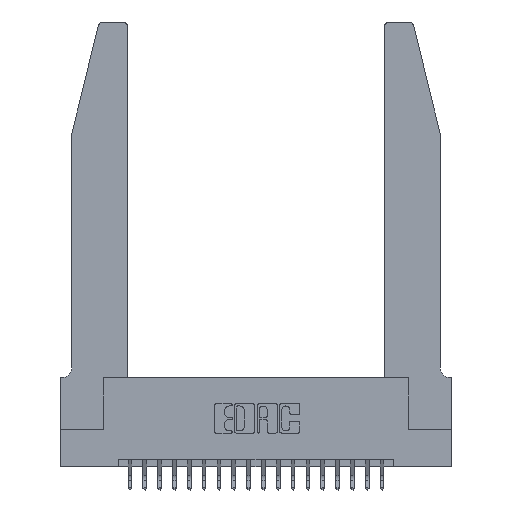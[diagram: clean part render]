
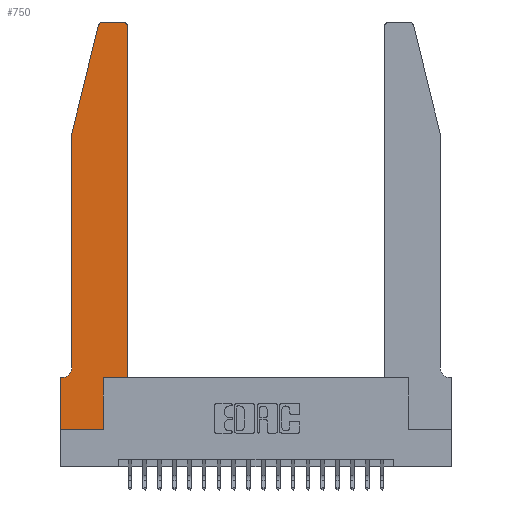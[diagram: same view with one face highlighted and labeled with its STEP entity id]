
A CAD part, top view. The second image highlights one B-rep face of the part: STEP entity #750.
In plain terms, the highlighted planar face has unit normal (0, 0, 1).
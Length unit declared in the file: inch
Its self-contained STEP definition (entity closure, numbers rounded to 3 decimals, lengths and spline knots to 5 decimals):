
#50 = VERTEX_POINT ( 'NONE', #18213 ) ;
#88 = ORIENTED_EDGE ( 'NONE', *, *, #21648, .T. ) ;
#132 = CARTESIAN_POINT ( 'NONE',  ( 0.2865, 0., 0.37 ) ) ;
#356 = LINE ( 'NONE', #10773, #19022 ) ;
#670 = CARTESIAN_POINT ( 'NONE',  ( 0.0755, 2., 0.37 ) ) ;
#750 = ADVANCED_FACE ( 'NONE', ( #14140 ), #21990, .T. ) ;
#799 = VERTEX_POINT ( 'NONE', #10004 ) ;
#1168 = LINE ( 'NONE', #1817, #9071 ) ;
#1387 = DIRECTION ( 'NONE',  ( 1., 0., 0. ) ) ;
#1817 = CARTESIAN_POINT ( 'NONE',  ( 0., 0., 0.37 ) ) ;
#1843 = CARTESIAN_POINT ( 'NONE',  ( 0.284, 2.75, 0.37 ) ) ;
#2261 = CIRCLE ( 'NONE', #8044, 0.03 ) ;
#2303 = VECTOR ( 'NONE', #19196, 39.37008 ) ;
#2811 = LINE ( 'NONE', #670, #19023 ) ;
#2984 = ORIENTED_EDGE ( 'NONE', *, *, #8302, .T. ) ;
#3949 = LINE ( 'NONE', #14047, #2303 ) ;
#4034 = DIRECTION ( 'NONE',  ( 1., 0., 0. ) ) ;
#4175 = CARTESIAN_POINT ( 'NONE',  ( 0., 0., 0.37 ) ) ;
#4612 = VERTEX_POINT ( 'NONE', #22006 ) ;
#4892 = EDGE_CURVE ( 'NONE', #15860, #11558, #11312, .T. ) ;
#5032 = ORIENTED_EDGE ( 'NONE', *, *, #19874, .T. ) ;
#5102 = EDGE_CURVE ( 'NONE', #50, #15860, #3949, .T. ) ;
#5191 = VECTOR ( 'NONE', #19702, 39.37008 ) ;
#5246 = CARTESIAN_POINT ( 'NONE',  ( 0.0755, 0.35, 0.37 ) ) ;
#5864 = LINE ( 'NONE', #14336, #19835 ) ;
#5895 = EDGE_CURVE ( 'NONE', #8026, #19718, #5864, .T. ) ;
#6040 = LINE ( 'NONE', #15882, #10870 ) ;
#6229 = EDGE_CURVE ( 'NONE', #10780, #50, #2261, .T. ) ;
#6900 = VERTEX_POINT ( 'NONE', #7355 ) ;
#7232 = CARTESIAN_POINT ( 'NONE',  ( 0.0055, 0.42, 0.37 ) ) ;
#7264 = CARTESIAN_POINT ( 'NONE',  ( 0., 0., 0.37 ) ) ;
#7355 = CARTESIAN_POINT ( 'NONE',  ( 0.0055, 0.35, 0.37 ) ) ;
#7405 = DIRECTION ( 'NONE',  ( 0., -1., 0. ) ) ;
#8026 = VERTEX_POINT ( 'NONE', #21622 ) ;
#8044 = AXIS2_PLACEMENT_3D ( 'NONE', #15621, #12115, #20733 ) ;
#8132 = LINE ( 'NONE', #7264, #21272 ) ;
#8302 = EDGE_CURVE ( 'NONE', #19718, #10780, #6040, .T. ) ;
#8345 = CARTESIAN_POINT ( 'NONE',  ( 0., 0.35, 0.37 ) ) ;
#8570 = LINE ( 'NONE', #5246, #20934 ) ;
#9071 = VECTOR ( 'NONE', #7405, 39.37008 ) ;
#9343 = CARTESIAN_POINT ( 'NONE',  ( 0.2865, 0.35, 0.37 ) ) ;
#10004 = CARTESIAN_POINT ( 'NONE',  ( 0.0755, 0.42, 0.37 ) ) ;
#10617 = ORIENTED_EDGE ( 'NONE', *, *, #4892, .T. ) ;
#10773 = CARTESIAN_POINT ( 'NONE',  ( 0.0755, 2., 0.37 ) ) ;
#10780 = VERTEX_POINT ( 'NONE', #20130 ) ;
#10870 = VECTOR ( 'NONE', #10917, 39.37008 ) ;
#10916 = DIRECTION ( 'NONE',  ( 0., 0., -1. ) ) ;
#10917 = DIRECTION ( 'NONE',  ( 0., 1., 0. ) ) ;
#10988 = DIRECTION ( 'NONE',  ( 0., -1., 0. ) ) ;
#11066 = ORIENTED_EDGE ( 'NONE', *, *, #14176, .T. ) ;
#11136 = CARTESIAN_POINT ( 'NONE',  ( 0.4505, 0.35, 0.37 ) ) ;
#11141 = LINE ( 'NONE', #9343, #5191 ) ;
#11235 = ORIENTED_EDGE ( 'NONE', *, *, #16200, .T. ) ;
#11312 = CIRCLE ( 'NONE', #20836, 0.03 ) ;
#11558 = VERTEX_POINT ( 'NONE', #15691 ) ;
#11735 = DIRECTION ( 'NONE',  ( 0., 0., 1. ) ) ;
#12115 = DIRECTION ( 'NONE',  ( 0., 0., 1. ) ) ;
#12174 = ORIENTED_EDGE ( 'NONE', *, *, #5102, .T. ) ;
#12661 = CARTESIAN_POINT ( 'NONE',  ( 0.284, 2.72, 0.37 ) ) ;
#12680 = EDGE_CURVE ( 'NONE', #799, #6900, #21186, .T. ) ;
#13039 = EDGE_CURVE ( 'NONE', #11558, #4612, #356, .T. ) ;
#13253 = EDGE_CURVE ( 'NONE', #14546, #18317, #1168, .T. ) ;
#13934 = AXIS2_PLACEMENT_3D ( 'NONE', #8345, #11735, #1387 ) ;
#14047 = CARTESIAN_POINT ( 'NONE',  ( 0.2605, 2.75, 0.37 ) ) ;
#14140 = FACE_OUTER_BOUND ( 'NONE', #17117, .T. ) ;
#14176 = EDGE_CURVE ( 'NONE', #4612, #799, #2811, .T. ) ;
#14185 = DIRECTION ( 'NONE',  ( 1., 0., 0. ) ) ;
#14336 = CARTESIAN_POINT ( 'NONE',  ( 0.4505, 0.35, 0.37 ) ) ;
#14401 = DIRECTION ( 'NONE',  ( 0., 0., 1. ) ) ;
#14546 = VERTEX_POINT ( 'NONE', #15054 ) ;
#15054 = CARTESIAN_POINT ( 'NONE',  ( 0., 0.35, 0.37 ) ) ;
#15621 = CARTESIAN_POINT ( 'NONE',  ( 0.4205, 2.72, 0.37 ) ) ;
#15691 = CARTESIAN_POINT ( 'NONE',  ( 0.25487, 2.72718, 0.37 ) ) ;
#15735 = DIRECTION ( 'NONE',  ( -0.239, -0.971, 0. ) ) ;
#15860 = VERTEX_POINT ( 'NONE', #1843 ) ;
#15882 = CARTESIAN_POINT ( 'NONE',  ( 0.4505, 0.35, 0.37 ) ) ;
#16166 = AXIS2_PLACEMENT_3D ( 'NONE', #7232, #10916, #19248 ) ;
#16200 = EDGE_CURVE ( 'NONE', #19452, #8026, #11141, .T. ) ;
#17117 = EDGE_LOOP ( 'NONE', ( #12174, #10617, #21827, #11066, #17355, #5032, #18017, #88, #11235, #17971, #2984, #20460 ) ) ;
#17355 = ORIENTED_EDGE ( 'NONE', *, *, #12680, .T. ) ;
#17971 = ORIENTED_EDGE ( 'NONE', *, *, #5895, .T. ) ;
#18017 = ORIENTED_EDGE ( 'NONE', *, *, #13253, .T. ) ;
#18213 = CARTESIAN_POINT ( 'NONE',  ( 0.4205, 2.75, 0.37 ) ) ;
#18317 = VERTEX_POINT ( 'NONE', #4175 ) ;
#19022 = VECTOR ( 'NONE', #15735, 39.37008 ) ;
#19023 = VECTOR ( 'NONE', #10988, 39.37008 ) ;
#19196 = DIRECTION ( 'NONE',  ( -1., 0., 0. ) ) ;
#19248 = DIRECTION ( 'NONE',  ( -1., 0., 0. ) ) ;
#19452 = VERTEX_POINT ( 'NONE', #132 ) ;
#19702 = DIRECTION ( 'NONE',  ( 0., 1., 0. ) ) ;
#19718 = VERTEX_POINT ( 'NONE', #11136 ) ;
#19835 = VECTOR ( 'NONE', #14185, 39.37008 ) ;
#19874 = EDGE_CURVE ( 'NONE', #6900, #14546, #8570, .T. ) ;
#20130 = CARTESIAN_POINT ( 'NONE',  ( 0.4505, 2.72, 0.37 ) ) ;
#20460 = ORIENTED_EDGE ( 'NONE', *, *, #6229, .T. ) ;
#20733 = DIRECTION ( 'NONE',  ( 1., 0., 0. ) ) ;
#20836 = AXIS2_PLACEMENT_3D ( 'NONE', #12661, #14401, #4034 ) ;
#20934 = VECTOR ( 'NONE', #21858, 39.37008 ) ;
#21186 = CIRCLE ( 'NONE', #16166, 0.07 ) ;
#21272 = VECTOR ( 'NONE', #21378, 39.37008 ) ;
#21378 = DIRECTION ( 'NONE',  ( 1., 0., 0. ) ) ;
#21622 = CARTESIAN_POINT ( 'NONE',  ( 0.2865, 0.35, 0.37 ) ) ;
#21648 = EDGE_CURVE ( 'NONE', #18317, #19452, #8132, .T. ) ;
#21827 = ORIENTED_EDGE ( 'NONE', *, *, #13039, .T. ) ;
#21858 = DIRECTION ( 'NONE',  ( -1., 0., 0. ) ) ;
#21990 = PLANE ( 'NONE',  #13934 ) ;
#22006 = CARTESIAN_POINT ( 'NONE',  ( 0.0755, 2., 0.37 ) ) ;
